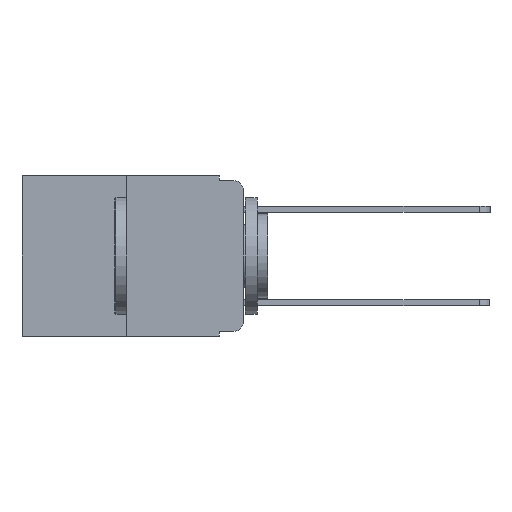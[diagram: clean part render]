
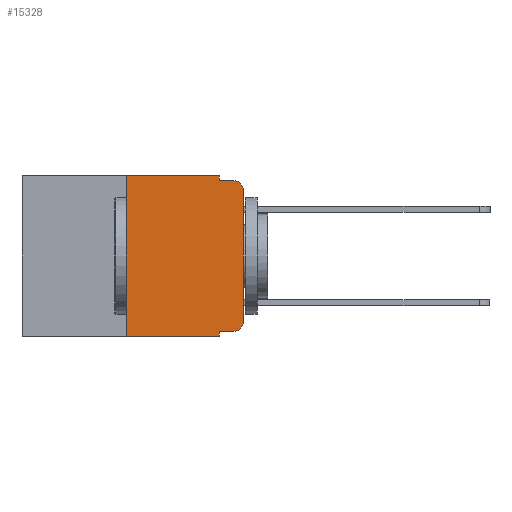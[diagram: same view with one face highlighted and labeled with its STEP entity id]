
A CAD part, left-side view. The second image highlights one B-rep face of the part: STEP entity #15328.
In plain terms, the highlighted planar face has unit normal (-1, 0, 0).
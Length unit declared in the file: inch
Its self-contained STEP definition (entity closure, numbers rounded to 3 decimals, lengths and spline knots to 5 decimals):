
#166 = EDGE_CURVE ( 'NONE', #1321, #1909, #14919, .T. ) ;
#252 = VERTEX_POINT ( 'NONE', #13182 ) ;
#533 = CARTESIAN_POINT ( 'NONE',  ( 0., 0., -0.313 ) ) ;
#1130 = PLANE ( 'NONE',  #11682 ) ;
#1155 = VERTEX_POINT ( 'NONE', #16554 ) ;
#1321 = VERTEX_POINT ( 'NONE', #8856 ) ;
#1333 = VECTOR ( 'NONE', #17806, 39.37008 ) ;
#1489 = EDGE_CURVE ( 'NONE', #1155, #20626, #3873, .T. ) ;
#1587 = ORIENTED_EDGE ( 'NONE', *, *, #19904, .T. ) ;
#1851 = VECTOR ( 'NONE', #20469, 39.37008 ) ;
#1909 = VERTEX_POINT ( 'NONE', #11095 ) ;
#2439 = ORIENTED_EDGE ( 'NONE', *, *, #6245, .T. ) ;
#2725 = EDGE_CURVE ( 'NONE', #6992, #16261, #12052, .T. ) ;
#2832 = CARTESIAN_POINT ( 'NONE',  ( 0., 0.25, 0. ) ) ;
#3008 = CARTESIAN_POINT ( 'NONE',  ( 0., 0., -0.03 ) ) ;
#3335 = DIRECTION ( 'NONE',  ( -1., 0., 0. ) ) ;
#3871 = CARTESIAN_POINT ( 'NONE',  ( 0., 0.473, -0.343 ) ) ;
#3873 = LINE ( 'NONE', #4394, #16712 ) ;
#3956 = EDGE_CURVE ( 'NONE', #16261, #14720, #7270, .T. ) ;
#4394 = CARTESIAN_POINT ( 'NONE',  ( 0., 0.25, 0. ) ) ;
#4772 = CARTESIAN_POINT ( 'NONE',  ( 0., 0.473, 0. ) ) ;
#5110 = EDGE_CURVE ( 'NONE', #19981, #14720, #16335, .T. ) ;
#5681 = DIRECTION ( 'NONE',  ( 0., -1., 0. ) ) ;
#5771 = ORIENTED_EDGE ( 'NONE', *, *, #20972, .T. ) ;
#6245 = EDGE_CURVE ( 'NONE', #13265, #19981, #6654, .T. ) ;
#6492 = DIRECTION ( 'NONE',  ( 0., 0., -1. ) ) ;
#6630 = CARTESIAN_POINT ( 'NONE',  ( 0., 0.473, 0. ) ) ;
#6654 = LINE ( 'NONE', #13706, #10599 ) ;
#6992 = VERTEX_POINT ( 'NONE', #18650 ) ;
#7094 = ORIENTED_EDGE ( 'NONE', *, *, #5110, .T. ) ;
#7140 = DIRECTION ( 'NONE',  ( 0., -1., 0. ) ) ;
#7270 = LINE ( 'NONE', #17083, #14513 ) ;
#7542 = EDGE_CURVE ( 'NONE', #20626, #6992, #10291, .T. ) ;
#7607 = ORIENTED_EDGE ( 'NONE', *, *, #2725, .F. ) ;
#8613 = EDGE_LOOP ( 'NONE', ( #2439, #7094, #15926, #7607, #8653, #13065, #9209, #13564, #5771, #1587 ) ) ;
#8653 = ORIENTED_EDGE ( 'NONE', *, *, #7542, .F. ) ;
#8856 = CARTESIAN_POINT ( 'NONE',  ( 0., 0.051, -0.333 ) ) ;
#9209 = ORIENTED_EDGE ( 'NONE', *, *, #15878, .T. ) ;
#9753 = CARTESIAN_POINT ( 'NONE',  ( 0., 0.051, 0. ) ) ;
#9784 = DIRECTION ( 'NONE',  ( -1., 0., 0. ) ) ;
#9785 = AXIS2_PLACEMENT_3D ( 'NONE', #13417, #3335, #15094 ) ;
#10037 = CARTESIAN_POINT ( 'NONE',  ( 0., 0.051, -0.01 ) ) ;
#10291 = LINE ( 'NONE', #6630, #18502 ) ;
#10599 = VECTOR ( 'NONE', #15409, 39.37008 ) ;
#10624 = DIRECTION ( 'NONE',  ( 0., -1., 0. ) ) ;
#10727 = CARTESIAN_POINT ( 'NONE',  ( 0., 0.051, 0. ) ) ;
#11095 = CARTESIAN_POINT ( 'NONE',  ( 0., 0.051, -0.343 ) ) ;
#11456 = AXIS2_PLACEMENT_3D ( 'NONE', #19559, #9784, #21163 ) ;
#11682 = AXIS2_PLACEMENT_3D ( 'NONE', #4772, #16466, #6492 ) ;
#12052 = LINE ( 'NONE', #10727, #1851 ) ;
#12551 = LINE ( 'NONE', #3871, #18457 ) ;
#13065 = ORIENTED_EDGE ( 'NONE', *, *, #1489, .F. ) ;
#13182 = CARTESIAN_POINT ( 'NONE',  ( 0., 0.02, -0.333 ) ) ;
#13265 = VERTEX_POINT ( 'NONE', #533 ) ;
#13280 = CARTESIAN_POINT ( 'NONE',  ( 0., 0.02, -0.01 ) ) ;
#13336 = VECTOR ( 'NONE', #5681, 39.37008 ) ;
#13417 = CARTESIAN_POINT ( 'NONE',  ( 0., 0.02, -0.03 ) ) ;
#13564 = ORIENTED_EDGE ( 'NONE', *, *, #166, .F. ) ;
#13706 = CARTESIAN_POINT ( 'NONE',  ( 0., 0., 0. ) ) ;
#14513 = VECTOR ( 'NONE', #7140, 39.37008 ) ;
#14720 = VERTEX_POINT ( 'NONE', #13280 ) ;
#14919 = LINE ( 'NONE', #9753, #1333 ) ;
#15094 = DIRECTION ( 'NONE',  ( 0., 0., -1. ) ) ;
#15328 = ADVANCED_FACE ( 'NONE', ( #21696 ), #1130, .F. ) ;
#15409 = DIRECTION ( 'NONE',  ( 0., 0., 1. ) ) ;
#15878 = EDGE_CURVE ( 'NONE', #1155, #1909, #12551, .T. ) ;
#15926 = ORIENTED_EDGE ( 'NONE', *, *, #3956, .F. ) ;
#16093 = DIRECTION ( 'NONE',  ( 0., 0., 1. ) ) ;
#16261 = VERTEX_POINT ( 'NONE', #10037 ) ;
#16335 = CIRCLE ( 'NONE', #9785, 0.02 ) ;
#16466 = DIRECTION ( 'NONE',  ( 1., 0., 0. ) ) ;
#16554 = CARTESIAN_POINT ( 'NONE',  ( 0., 0.25, -0.343 ) ) ;
#16712 = VECTOR ( 'NONE', #16093, 39.37008 ) ;
#17083 = CARTESIAN_POINT ( 'NONE',  ( 0., 0.051, -0.01 ) ) ;
#17287 = CIRCLE ( 'NONE', #11456, 0.02 ) ;
#17323 = CARTESIAN_POINT ( 'NONE',  ( 0., 0.051, -0.333 ) ) ;
#17741 = LINE ( 'NONE', #17323, #13336 ) ;
#17806 = DIRECTION ( 'NONE',  ( 0., 0., -1. ) ) ;
#18457 = VECTOR ( 'NONE', #10624, 39.37008 ) ;
#18502 = VECTOR ( 'NONE', #19801, 39.37008 ) ;
#18650 = CARTESIAN_POINT ( 'NONE',  ( 0., 0.051, 0. ) ) ;
#19559 = CARTESIAN_POINT ( 'NONE',  ( 0., 0.02, -0.313 ) ) ;
#19801 = DIRECTION ( 'NONE',  ( 0., -1., 0. ) ) ;
#19904 = EDGE_CURVE ( 'NONE', #252, #13265, #17287, .T. ) ;
#19981 = VERTEX_POINT ( 'NONE', #3008 ) ;
#20469 = DIRECTION ( 'NONE',  ( 0., 0., -1. ) ) ;
#20626 = VERTEX_POINT ( 'NONE', #2832 ) ;
#20972 = EDGE_CURVE ( 'NONE', #1321, #252, #17741, .T. ) ;
#21163 = DIRECTION ( 'NONE',  ( 0., 0., -1. ) ) ;
#21696 = FACE_OUTER_BOUND ( 'NONE', #8613, .T. ) ;
